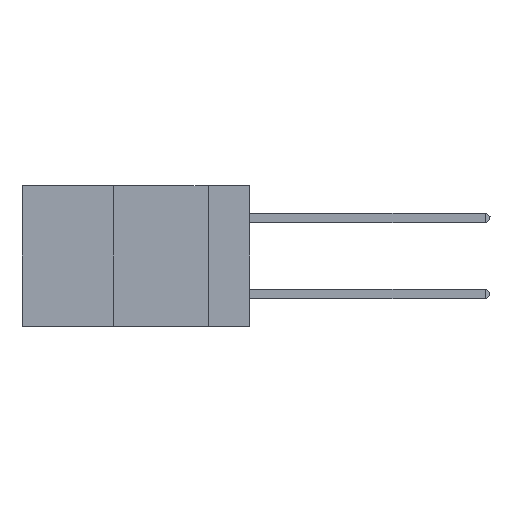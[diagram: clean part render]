
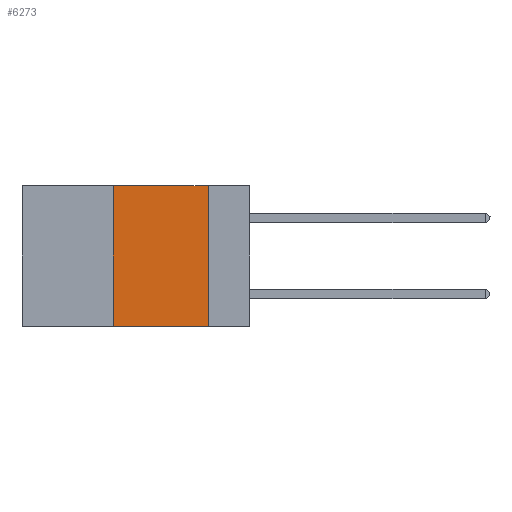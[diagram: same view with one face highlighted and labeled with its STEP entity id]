
A CAD part, left-side view. The second image highlights one B-rep face of the part: STEP entity #6273.
In plain terms, the highlighted planar face has unit normal (-1, 0, 0).
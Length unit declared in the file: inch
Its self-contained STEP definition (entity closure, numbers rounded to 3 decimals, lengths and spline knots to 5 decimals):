
#164 = VECTOR ( 'NONE', #7641, 39.37008 ) ;
#175 = LINE ( 'NONE', #6951, #2700 ) ;
#247 = CARTESIAN_POINT ( 'NONE',  ( 0., 0.6, 0. ) ) ;
#633 = VERTEX_POINT ( 'NONE', #4301 ) ;
#672 = DIRECTION ( 'NONE',  ( 0., 0., 1. ) ) ;
#1700 = EDGE_CURVE ( 'NONE', #633, #12641, #12478, .T. ) ;
#2118 = PLANE ( 'NONE',  #6793 ) ;
#2360 = EDGE_CURVE ( 'NONE', #6871, #4802, #175, .T. ) ;
#2666 = LINE ( 'NONE', #3560, #164 ) ;
#2700 = VECTOR ( 'NONE', #11989, 39.37008 ) ;
#2827 = LINE ( 'NONE', #12560, #11584 ) ;
#3005 = DIRECTION ( 'NONE',  ( 0., -1., 0. ) ) ;
#3560 = CARTESIAN_POINT ( 'NONE',  ( 0., 0.6, 0. ) ) ;
#4301 = CARTESIAN_POINT ( 'NONE',  ( 0., 0.36, -0.37 ) ) ;
#4796 = EDGE_CURVE ( 'NONE', #12641, #6871, #2666, .T. ) ;
#4802 = VERTEX_POINT ( 'NONE', #11582 ) ;
#4806 = EDGE_LOOP ( 'NONE', ( #5091, #10879, #9563, #4875 ) ) ;
#4875 = ORIENTED_EDGE ( 'NONE', *, *, #9187, .T. ) ;
#4898 = CARTESIAN_POINT ( 'NONE',  ( 0., 0.36, 0. ) ) ;
#5091 = ORIENTED_EDGE ( 'NONE', *, *, #2360, .F. ) ;
#6051 = DIRECTION ( 'NONE',  ( 1., 0., 0. ) ) ;
#6273 = ADVANCED_FACE ( 'NONE', ( #7147 ), #2118, .F. ) ;
#6793 = AXIS2_PLACEMENT_3D ( 'NONE', #247, #6051, #10110 ) ;
#6871 = VERTEX_POINT ( 'NONE', #7438 ) ;
#6951 = CARTESIAN_POINT ( 'NONE',  ( 0., 0.11, 0. ) ) ;
#7147 = FACE_OUTER_BOUND ( 'NONE', #4806, .T. ) ;
#7438 = CARTESIAN_POINT ( 'NONE',  ( 0., 0.11, 0. ) ) ;
#7641 = DIRECTION ( 'NONE',  ( 0., -1., 0. ) ) ;
#7776 = CARTESIAN_POINT ( 'NONE',  ( 0., 0.36, 0. ) ) ;
#8908 = VECTOR ( 'NONE', #672, 39.37008 ) ;
#9187 = EDGE_CURVE ( 'NONE', #633, #4802, #2827, .T. ) ;
#9563 = ORIENTED_EDGE ( 'NONE', *, *, #1700, .F. ) ;
#10110 = DIRECTION ( 'NONE',  ( 0., 0., -1. ) ) ;
#10879 = ORIENTED_EDGE ( 'NONE', *, *, #4796, .F. ) ;
#11582 = CARTESIAN_POINT ( 'NONE',  ( 0., 0.11, -0.37 ) ) ;
#11584 = VECTOR ( 'NONE', #3005, 39.37008 ) ;
#11989 = DIRECTION ( 'NONE',  ( 0., 0., -1. ) ) ;
#12478 = LINE ( 'NONE', #7776, #8908 ) ;
#12560 = CARTESIAN_POINT ( 'NONE',  ( 0., 0.6, -0.37 ) ) ;
#12641 = VERTEX_POINT ( 'NONE', #4898 ) ;
